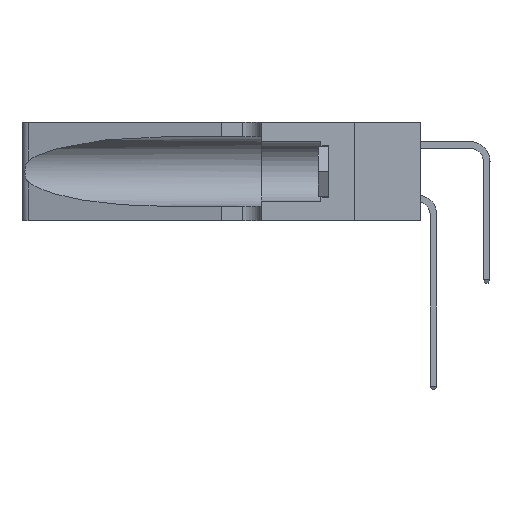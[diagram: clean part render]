
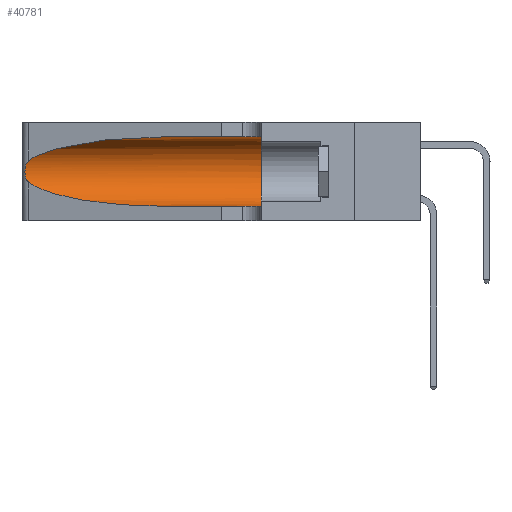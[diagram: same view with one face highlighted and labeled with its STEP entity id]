
A CAD part, left-side view. The second image highlights one B-rep face of the part: STEP entity #40781.
In plain terms, the highlighted cylindrical face has radius 3.308 mm (diameter 6.617 mm), a partial arc.
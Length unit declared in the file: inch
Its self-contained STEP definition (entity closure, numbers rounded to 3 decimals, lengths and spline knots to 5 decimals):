
#332 = CARTESIAN_POINT ( 'NONE',  ( 0.25787, 1.23484, 0.2124 ) ) ;
#2186 = EDGE_CURVE ( 'NONE', #34630, #24870, #36178, .T. ) ;
#2219 = DIRECTION ( 'NONE',  ( 0., 1., 0. ) ) ;
#2536 = CARTESIAN_POINT ( 'NONE',  ( 0.1305, 0.72297, 0.31525 ) ) ;
#3448 = EDGE_CURVE ( 'NONE', #8217, #5437, #28735, .T. ) ;
#4644 = ORIENTED_EDGE ( 'NONE', *, *, #2186, .T. ) ;
#4955 = DIRECTION ( 'NONE',  ( 0., -1., 0. ) ) ;
#5415 = DIRECTION ( 'NONE',  ( 0., 0., 1. ) ) ;
#5437 = VERTEX_POINT ( 'NONE', #32661 ) ;
#6542 = ORIENTED_EDGE ( 'NONE', *, *, #14035, .T. ) ;
#6714 = CYLINDRICAL_SURFACE ( 'NONE', #41498, 0.13025 ) ;
#6819 = CARTESIAN_POINT ( 'NONE',  ( 0.26018, 1.23835, 0.19895 ) ) ;
#7276 = VERTEX_POINT ( 'NONE', #29430 ) ;
#8217 = VERTEX_POINT ( 'NONE', #15593 ) ;
#8265 = EDGE_CURVE ( 'NONE', #9290, #34630, #35683, .T. ) ;
#8976 = VECTOR ( 'NONE', #33537, 39.37008 ) ;
#9088 = CARTESIAN_POINT ( 'NONE',  ( 0.2373, 1.15595, 0.08982 ) ) ;
#9290 = VERTEX_POINT ( 'NONE', #20854 ) ;
#10084 = CARTESIAN_POINT ( 'NONE',  ( 0.26075, 1.23896, 0.19203 ) ) ;
#10219 = CARTESIAN_POINT ( 'NONE',  ( 0.25639, 1.23184, 0.21858 ) ) ;
#10930 = CARTESIAN_POINT ( 'NONE',  ( 0.25789, 1.23486, 0.15765 ) ) ;
#12161 = EDGE_CURVE ( 'NONE', #9290, #8217, #26898, .T. ) ;
#13338 = CARTESIAN_POINT ( 'NONE',  ( 0.26075, 1.23896, 0.178 ) ) ;
#14018 = LINE ( 'NONE', #39435, #8976 ) ;
#14035 = EDGE_CURVE ( 'NONE', #24870, #7276, #34425, .T. ) ;
#15593 = CARTESIAN_POINT ( 'NONE',  ( 0.1305, 0.35, 0.31525 ) ) ;
#15609 = CARTESIAN_POINT ( 'NONE',  ( 0.1305, 0.72297, 0.05475 ) ) ;
#15772 = CARTESIAN_POINT ( 'NONE',  ( 0.18966, 0.96281, 0.31525 ) ) ;
#16582 = CARTESIAN_POINT ( 'NONE',  ( 0.2373, 1.15595, 0.28018 ) ) ;
#16875 = CARTESIAN_POINT ( 'NONE',  ( 0.25555, 1.22993, 0.14849 ) ) ;
#17674 = VECTOR ( 'NONE', #4955, 39.37008 ) ;
#18053 = EDGE_CURVE ( 'NONE', #7276, #5437, #14018, .T. ) ;
#18160 = CARTESIAN_POINT ( 'NONE',  ( 0.25487, 1.22718, 0.14631 ) ) ;
#20445 = CARTESIAN_POINT ( 'NONE',  ( 0.25487, 1.22718, 0.22369 ) ) ;
#20854 = CARTESIAN_POINT ( 'NONE',  ( 0.1305, 0.72297, 0.31525 ) ) ;
#23025 = CARTESIAN_POINT ( 'NONE',  ( 0.25487, 1.22718, 0.22369 ) ) ;
#24870 = VERTEX_POINT ( 'NONE', #41367 ) ;
#26085 = FACE_OUTER_BOUND ( 'NONE', #27510, .T. ) ;
#26205 = CARTESIAN_POINT ( 'NONE',  ( 0.25487, 1.22718, 0.22369 ) ) ;
#26339 = CARTESIAN_POINT ( 'NONE',  ( 0.25854, 1.2359, 0.20912 ) ) ;
#26599 = CARTESIAN_POINT ( 'NONE',  ( 0.25487, 1.22718, 0.14631 ) ) ;
#26880 = CARTESIAN_POINT ( 'NONE',  ( 0.25856, 1.23593, 0.16098 ) ) ;
#26898 = LINE ( 'NONE', #27009, #17674 ) ;
#27009 = CARTESIAN_POINT ( 'NONE',  ( 0.1305, 1.61858, 0.31525 ) ) ;
#27018 = CARTESIAN_POINT ( 'NONE',  ( 0.25639, 1.23186, 0.15144 ) ) ;
#27171 = CARTESIAN_POINT ( 'NONE',  ( 0.26017, 1.23833, 0.17102 ) ) ;
#27510 = EDGE_LOOP ( 'NONE', ( #31389, #4644, #6542, #35778, #32939, #31020 ) ) ;
#28735 = CIRCLE ( 'NONE', #40913, 0.13025 ) ;
#29430 = CARTESIAN_POINT ( 'NONE',  ( 0.1305, 0.72297, 0.05475 ) ) ;
#31020 = ORIENTED_EDGE ( 'NONE', *, *, #12161, .F. ) ;
#31389 = ORIENTED_EDGE ( 'NONE', *, *, #8265, .T. ) ;
#31880 = CARTESIAN_POINT ( 'NONE',  ( 0.18966, 0.96281, 0.05475 ) ) ;
#32661 = CARTESIAN_POINT ( 'NONE',  ( 0.1305, 0.35, 0.05475 ) ) ;
#32939 = ORIENTED_EDGE ( 'NONE', *, *, #3448, .F. ) ;
#33537 = DIRECTION ( 'NONE',  ( 0., -1., 0. ) ) ;
#34425 =( BOUNDED_CURVE ( )  B_SPLINE_CURVE ( 3, ( #18160, #9088, #31880, #15609 ),
 .UNSPECIFIED., .F., .F. ) 
 B_SPLINE_CURVE_WITH_KNOTS ( ( 4, 4 ),
 ( 3.44316, 4.71239 ),
 .UNSPECIFIED. ) 
 CURVE ( )  GEOMETRIC_REPRESENTATION_ITEM ( )  RATIONAL_B_SPLINE_CURVE ( ( 1., 0.87, 0.87, 1. ) ) 
 REPRESENTATION_ITEM ( '' )  );
#34630 = VERTEX_POINT ( 'NONE', #23025 ) ;
#34826 = CARTESIAN_POINT ( 'NONE',  ( 0.1305, 0.35, 0.185 ) ) ;
#35683 =( BOUNDED_CURVE ( )  B_SPLINE_CURVE ( 3, ( #2536, #15772, #16582, #20445 ),
 .UNSPECIFIED., .F., .F. ) 
 B_SPLINE_CURVE_WITH_KNOTS ( ( 4, 4 ),
 ( 1.5708, 2.84003 ),
 .UNSPECIFIED. ) 
 CURVE ( )  GEOMETRIC_REPRESENTATION_ITEM ( )  RATIONAL_B_SPLINE_CURVE ( ( 1., 0.87, 0.87, 1. ) ) 
 REPRESENTATION_ITEM ( '' )  );
#35778 = ORIENTED_EDGE ( 'NONE', *, *, #18053, .T. ) ;
#36178 = B_SPLINE_CURVE_WITH_KNOTS ( 'NONE', 3,
 ( #26205, #39174, #10219, #332, #26339, #6819, #10084, #13338, #27171, #26880, #10930, #27018, #16875, #26599 ),
 .UNSPECIFIED., .F., .F.,
 ( 4, 2, 2, 2, 2, 2, 4 ),
 ( 0., 0.00027, 0.00053, 0.00107, 0.0016, 0.00187, 0.00214 ),
 .UNSPECIFIED. ) ;
#38048 = DIRECTION ( 'NONE',  ( 0., -1., 0. ) ) ;
#38329 = CARTESIAN_POINT ( 'NONE',  ( 0.1305, 1.61858, 0.185 ) ) ;
#39174 = CARTESIAN_POINT ( 'NONE',  ( 0.25555, 1.22994, 0.2215 ) ) ;
#39435 = CARTESIAN_POINT ( 'NONE',  ( 0.1305, 1.61858, 0.05475 ) ) ;
#40781 = ADVANCED_FACE ( 'NONE', ( #26085 ), #6714, .F. ) ;
#40913 = AXIS2_PLACEMENT_3D ( 'NONE', #34826, #2219, #5415 ) ;
#41367 = CARTESIAN_POINT ( 'NONE',  ( 0.25487, 1.22718, 0.14631 ) ) ;
#41483 = DIRECTION ( 'NONE',  ( 0., 0., -1. ) ) ;
#41498 = AXIS2_PLACEMENT_3D ( 'NONE', #38329, #38048, #41483 ) ;
